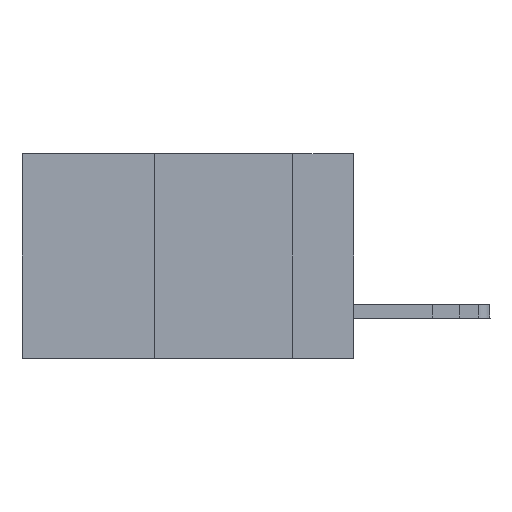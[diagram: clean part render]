
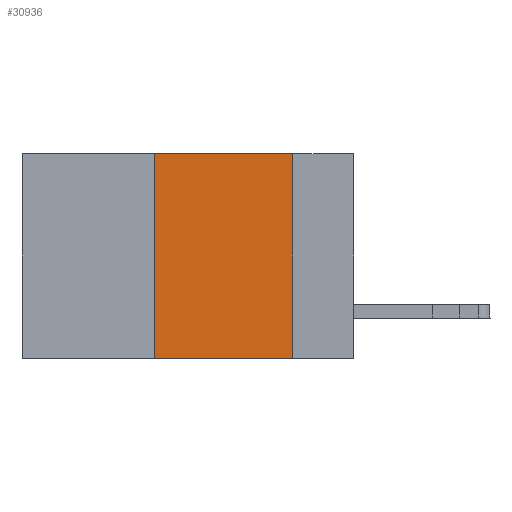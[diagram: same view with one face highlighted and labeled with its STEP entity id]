
A CAD part, left-side view. The second image highlights one B-rep face of the part: STEP entity #30936.
In plain terms, the highlighted planar face has unit normal (-1, 0, 0).
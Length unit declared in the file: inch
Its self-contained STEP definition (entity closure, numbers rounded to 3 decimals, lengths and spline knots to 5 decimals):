
#123 = DIRECTION ( 'NONE',  ( 0., -1., 0. ) ) ;
#3966 = DIRECTION ( 'NONE',  ( 0., 0., -1. ) ) ;
#4955 = LINE ( 'NONE', #20832, #36038 ) ;
#6600 = PLANE ( 'NONE',  #16942 ) ;
#7244 = LINE ( 'NONE', #18294, #32169 ) ;
#8382 = DIRECTION ( 'NONE',  ( 0., -1., 0. ) ) ;
#8478 = VECTOR ( 'NONE', #3966, 39.37008 ) ;
#11346 = ORIENTED_EDGE ( 'NONE', *, *, #12548, .T. ) ;
#12548 = EDGE_CURVE ( 'NONE', #16931, #34196, #31959, .T. ) ;
#15703 = DIRECTION ( 'NONE',  ( 0., 0., -1. ) ) ;
#15965 = CARTESIAN_POINT ( 'NONE',  ( 0., 0.36, -0.37 ) ) ;
#16069 = ORIENTED_EDGE ( 'NONE', *, *, #35208, .F. ) ;
#16931 = VERTEX_POINT ( 'NONE', #15965 ) ;
#16942 = AXIS2_PLACEMENT_3D ( 'NONE', #24647, #33674, #15703 ) ;
#17331 = CARTESIAN_POINT ( 'NONE',  ( 0., 0.6, -0.37 ) ) ;
#18294 = CARTESIAN_POINT ( 'NONE',  ( 0., 0.6, 0. ) ) ;
#19056 = CARTESIAN_POINT ( 'NONE',  ( 0., 0.11, 0. ) ) ;
#19456 = VERTEX_POINT ( 'NONE', #25333 ) ;
#20093 = EDGE_LOOP ( 'NONE', ( #20539, #25677, #16069, #11346 ) ) ;
#20539 = ORIENTED_EDGE ( 'NONE', *, *, #26451, .F. ) ;
#20832 = CARTESIAN_POINT ( 'NONE',  ( 0., 0.36, 0. ) ) ;
#21152 = CARTESIAN_POINT ( 'NONE',  ( 0., 0.36, 0. ) ) ;
#23897 = DIRECTION ( 'NONE',  ( 0., 0., 1. ) ) ;
#24017 = VECTOR ( 'NONE', #8382, 39.37008 ) ;
#24497 = LINE ( 'NONE', #19056, #8478 ) ;
#24647 = CARTESIAN_POINT ( 'NONE',  ( 0., 0.6, 0. ) ) ;
#25333 = CARTESIAN_POINT ( 'NONE',  ( 0., 0.11, 0. ) ) ;
#25677 = ORIENTED_EDGE ( 'NONE', *, *, #31380, .F. ) ;
#26451 = EDGE_CURVE ( 'NONE', #19456, #34196, #24497, .T. ) ;
#29537 = VERTEX_POINT ( 'NONE', #21152 ) ;
#30746 = CARTESIAN_POINT ( 'NONE',  ( 0., 0.11, -0.37 ) ) ;
#30936 = ADVANCED_FACE ( 'NONE', ( #31275 ), #6600, .F. ) ;
#31275 = FACE_OUTER_BOUND ( 'NONE', #20093, .T. ) ;
#31380 = EDGE_CURVE ( 'NONE', #29537, #19456, #7244, .T. ) ;
#31959 = LINE ( 'NONE', #17331, #24017 ) ;
#32169 = VECTOR ( 'NONE', #123, 39.37008 ) ;
#33674 = DIRECTION ( 'NONE',  ( 1., 0., 0. ) ) ;
#34196 = VERTEX_POINT ( 'NONE', #30746 ) ;
#35208 = EDGE_CURVE ( 'NONE', #16931, #29537, #4955, .T. ) ;
#36038 = VECTOR ( 'NONE', #23897, 39.37008 ) ;
